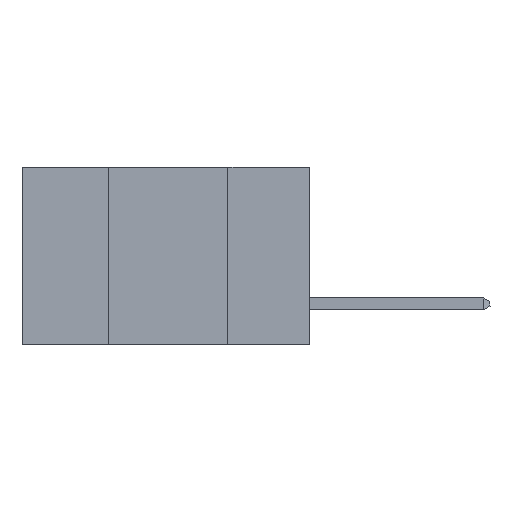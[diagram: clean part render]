
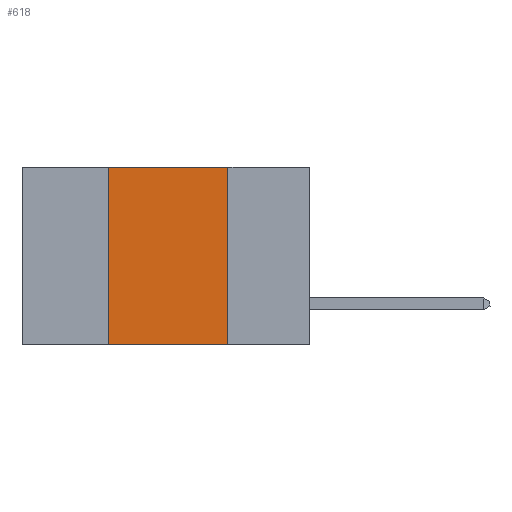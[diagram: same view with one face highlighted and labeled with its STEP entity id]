
A CAD part, left-side view. The second image highlights one B-rep face of the part: STEP entity #618.
In plain terms, the highlighted planar face has unit normal (-1, 0, 0).
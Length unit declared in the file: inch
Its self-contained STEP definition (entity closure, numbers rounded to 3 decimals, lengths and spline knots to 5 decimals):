
#110 = LINE ( 'NONE', #19424, #16316 ) ;
#228 = VERTEX_POINT ( 'NONE', #17298 ) ;
#618 = ADVANCED_FACE ( 'NONE', ( #9242 ), #18643, .F. ) ;
#1329 = VECTOR ( 'NONE', #23123, 39.37008 ) ;
#2305 = EDGE_CURVE ( 'NONE', #2714, #24797, #7360, .T. ) ;
#2516 = ORIENTED_EDGE ( 'NONE', *, *, #13580, .F. ) ;
#2714 = VERTEX_POINT ( 'NONE', #20874 ) ;
#2731 = DIRECTION ( 'NONE',  ( 1., 0., 0. ) ) ;
#4474 = EDGE_LOOP ( 'NONE', ( #22462, #2516, #8371, #13532 ) ) ;
#4778 = LINE ( 'NONE', #11699, #1329 ) ;
#7360 = LINE ( 'NONE', #8645, #11903 ) ;
#7571 = CARTESIAN_POINT ( 'NONE',  ( 0., 0.6, 0. ) ) ;
#7915 = DIRECTION ( 'NONE',  ( 0., 0., 1. ) ) ;
#7992 = DIRECTION ( 'NONE',  ( 0., -1., 0. ) ) ;
#8371 = ORIENTED_EDGE ( 'NONE', *, *, #22999, .F. ) ;
#8645 = CARTESIAN_POINT ( 'NONE',  ( 0., 0.6, -0.37 ) ) ;
#8679 = DIRECTION ( 'NONE',  ( 0., -1., 0. ) ) ;
#9242 = FACE_OUTER_BOUND ( 'NONE', #4474, .T. ) ;
#10187 = VERTEX_POINT ( 'NONE', #13034 ) ;
#10926 = AXIS2_PLACEMENT_3D ( 'NONE', #7571, #2731, #18664 ) ;
#11245 = LINE ( 'NONE', #16379, #20839 ) ;
#11699 = CARTESIAN_POINT ( 'NONE',  ( 0., 0.17, 0. ) ) ;
#11903 = VECTOR ( 'NONE', #7992, 39.37008 ) ;
#13034 = CARTESIAN_POINT ( 'NONE',  ( 0., 0.42, 0. ) ) ;
#13532 = ORIENTED_EDGE ( 'NONE', *, *, #2305, .T. ) ;
#13580 = EDGE_CURVE ( 'NONE', #10187, #228, #11245, .T. ) ;
#16316 = VECTOR ( 'NONE', #7915, 39.37008 ) ;
#16379 = CARTESIAN_POINT ( 'NONE',  ( 0., 0.6, 0. ) ) ;
#17298 = CARTESIAN_POINT ( 'NONE',  ( 0., 0.17, 0. ) ) ;
#17657 = CARTESIAN_POINT ( 'NONE',  ( 0., 0.17, -0.37 ) ) ;
#18643 = PLANE ( 'NONE',  #10926 ) ;
#18664 = DIRECTION ( 'NONE',  ( 0., 0., -1. ) ) ;
#19424 = CARTESIAN_POINT ( 'NONE',  ( 0., 0.42, 0. ) ) ;
#19671 = EDGE_CURVE ( 'NONE', #228, #24797, #4778, .T. ) ;
#20839 = VECTOR ( 'NONE', #8679, 39.37008 ) ;
#20874 = CARTESIAN_POINT ( 'NONE',  ( 0., 0.42, -0.37 ) ) ;
#22462 = ORIENTED_EDGE ( 'NONE', *, *, #19671, .F. ) ;
#22999 = EDGE_CURVE ( 'NONE', #2714, #10187, #110, .T. ) ;
#23123 = DIRECTION ( 'NONE',  ( 0., 0., -1. ) ) ;
#24797 = VERTEX_POINT ( 'NONE', #17657 ) ;
